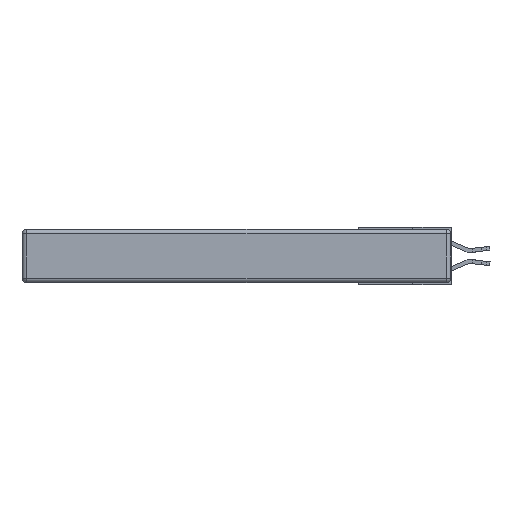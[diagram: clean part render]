
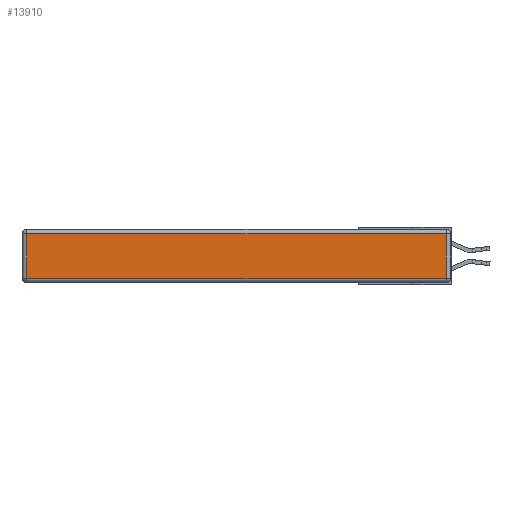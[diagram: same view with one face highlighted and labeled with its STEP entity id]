
A CAD part, left-side view. The second image highlights one B-rep face of the part: STEP entity #13910.
In plain terms, the highlighted planar face has unit normal (-1, 0, 0).
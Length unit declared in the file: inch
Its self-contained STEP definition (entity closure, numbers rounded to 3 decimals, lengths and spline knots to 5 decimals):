
#166 = CARTESIAN_POINT ( 'NONE',  ( 0., 2.72, -0.03 ) ) ;
#1098 = DIRECTION ( 'NONE',  ( 0., 0., 1. ) ) ;
#1977 = CARTESIAN_POINT ( 'NONE',  ( 0., 0., -0.313 ) ) ;
#2238 = CARTESIAN_POINT ( 'NONE',  ( 0., 2.75, -0.03 ) ) ;
#2286 = EDGE_CURVE ( 'NONE', #10572, #7529, #11452, .T. ) ;
#3306 = CARTESIAN_POINT ( 'NONE',  ( 0., 0.03, -0.343 ) ) ;
#4043 = CARTESIAN_POINT ( 'NONE',  ( 0., 0.03, -0.03 ) ) ;
#4159 = ORIENTED_EDGE ( 'NONE', *, *, #17584, .T. ) ;
#4184 = VECTOR ( 'NONE', #17537, 39.37008 ) ;
#4368 = DIRECTION ( 'NONE',  ( -1., 0., 0. ) ) ;
#4589 = LINE ( 'NONE', #3306, #17943 ) ;
#6478 = AXIS2_PLACEMENT_3D ( 'NONE', #21546, #4368, #1098 ) ;
#7529 = VERTEX_POINT ( 'NONE', #11859 ) ;
#7560 = CARTESIAN_POINT ( 'NONE',  ( 0., 2.72, -0.313 ) ) ;
#8750 = VECTOR ( 'NONE', #15799, 39.37008 ) ;
#10218 = DIRECTION ( 'NONE',  ( 0., 0., 1. ) ) ;
#10353 = FACE_OUTER_BOUND ( 'NONE', #15501, .T. ) ;
#10572 = VERTEX_POINT ( 'NONE', #7560 ) ;
#11138 = LINE ( 'NONE', #12534, #20736 ) ;
#11452 = LINE ( 'NONE', #1977, #8750 ) ;
#11859 = CARTESIAN_POINT ( 'NONE',  ( 0., 0.03, -0.313 ) ) ;
#12034 = VERTEX_POINT ( 'NONE', #166 ) ;
#12514 = ORIENTED_EDGE ( 'NONE', *, *, #2286, .T. ) ;
#12534 = CARTESIAN_POINT ( 'NONE',  ( 0., 2.72, -0.343 ) ) ;
#12953 = PLANE ( 'NONE',  #6478 ) ;
#13520 = EDGE_CURVE ( 'NONE', #21248, #12034, #14895, .T. ) ;
#13574 = EDGE_CURVE ( 'NONE', #12034, #10572, #11138, .T. ) ;
#13910 = ADVANCED_FACE ( 'NONE', ( #10353 ), #12953, .T. ) ;
#14895 = LINE ( 'NONE', #2238, #4184 ) ;
#14951 = ORIENTED_EDGE ( 'NONE', *, *, #13574, .T. ) ;
#15501 = EDGE_LOOP ( 'NONE', ( #12514, #4159, #21378, #14951 ) ) ;
#15799 = DIRECTION ( 'NONE',  ( 0., -1., 0. ) ) ;
#17537 = DIRECTION ( 'NONE',  ( 0., 1., 0. ) ) ;
#17584 = EDGE_CURVE ( 'NONE', #7529, #21248, #4589, .T. ) ;
#17943 = VECTOR ( 'NONE', #10218, 39.37008 ) ;
#20736 = VECTOR ( 'NONE', #21095, 39.37008 ) ;
#21095 = DIRECTION ( 'NONE',  ( 0., 0., -1. ) ) ;
#21248 = VERTEX_POINT ( 'NONE', #4043 ) ;
#21378 = ORIENTED_EDGE ( 'NONE', *, *, #13520, .T. ) ;
#21546 = CARTESIAN_POINT ( 'NONE',  ( 0., 0., -0.343 ) ) ;
